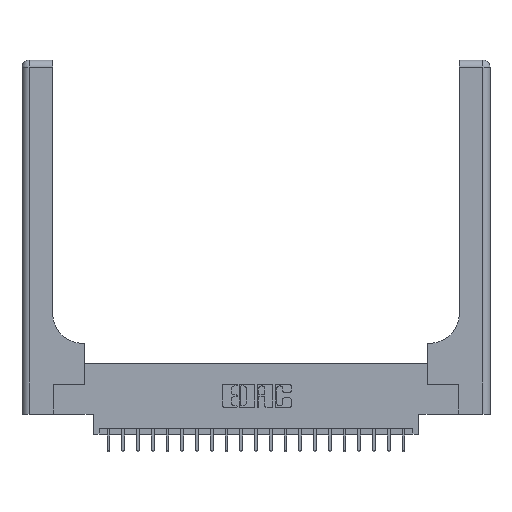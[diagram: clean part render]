
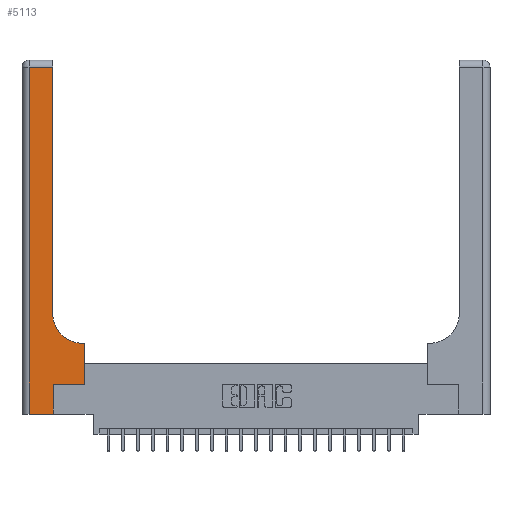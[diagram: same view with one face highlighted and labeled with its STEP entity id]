
A CAD part, top view. The second image highlights one B-rep face of the part: STEP entity #5113.
In plain terms, the highlighted planar face has unit normal (0, 0, 1).
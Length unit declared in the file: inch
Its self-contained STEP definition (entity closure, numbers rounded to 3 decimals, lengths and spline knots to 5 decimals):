
#341 = EDGE_CURVE ( 'NONE', #14062, #20262, #6236, .T. ) ;
#424 = ORIENTED_EDGE ( 'NONE', *, *, #341, .T. ) ;
#533 = LINE ( 'NONE', #12479, #3521 ) ;
#1240 = ORIENTED_EDGE ( 'NONE', *, *, #5312, .T. ) ;
#1293 = DIRECTION ( 'NONE',  ( -1., 0., 0. ) ) ;
#1605 = VECTOR ( 'NONE', #18984, 39.37008 ) ;
#1949 = EDGE_CURVE ( 'NONE', #20262, #14059, #13385, .T. ) ;
#2393 = VERTEX_POINT ( 'NONE', #12320 ) ;
#2599 = VECTOR ( 'NONE', #13983, 39.37008 ) ;
#3425 = ORIENTED_EDGE ( 'NONE', *, *, #14612, .T. ) ;
#3521 = VECTOR ( 'NONE', #17508, 39.37008 ) ;
#3938 = VERTEX_POINT ( 'NONE', #20074 ) ;
#5113 = ADVANCED_FACE ( 'NONE', ( #10994 ), #8161, .F. ) ;
#5312 = EDGE_CURVE ( 'NONE', #14059, #14385, #15191, .T. ) ;
#5616 = CARTESIAN_POINT ( 'NONE',  ( 0.26, 0.85, 0.37 ) ) ;
#6206 = DIRECTION ( 'NONE',  ( 0., -1., 0. ) ) ;
#6236 = LINE ( 'NONE', #7893, #15282 ) ;
#6695 = DIRECTION ( 'NONE',  ( 0., 1., 0. ) ) ;
#7032 = CARTESIAN_POINT ( 'NONE',  ( 0.51, 0.6, 0.37 ) ) ;
#7867 = DIRECTION ( 'NONE',  ( -1., 0., 0. ) ) ;
#7893 = CARTESIAN_POINT ( 'NONE',  ( 0., 2.94, 0.37 ) ) ;
#8161 = PLANE ( 'NONE',  #11349 ) ;
#8549 = CARTESIAN_POINT ( 'NONE',  ( 0.51, 0.85, 0.37 ) ) ;
#8555 = ORIENTED_EDGE ( 'NONE', *, *, #16205, .T. ) ;
#8695 = CARTESIAN_POINT ( 'NONE',  ( 0.528, 0.6, 0.37 ) ) ;
#9153 = LINE ( 'NONE', #20043, #21865 ) ;
#9530 = CARTESIAN_POINT ( 'NONE',  ( 0.06, 2.94, 0.37 ) ) ;
#9998 = LINE ( 'NONE', #15172, #18344 ) ;
#10207 = ORIENTED_EDGE ( 'NONE', *, *, #14818, .T. ) ;
#10309 = DIRECTION ( 'NONE',  ( 1., 0., 0. ) ) ;
#10994 = FACE_OUTER_BOUND ( 'NONE', #13477, .T. ) ;
#11235 = LINE ( 'NONE', #11469, #19562 ) ;
#11349 = AXIS2_PLACEMENT_3D ( 'NONE', #21504, #11626, #1293 ) ;
#11469 = CARTESIAN_POINT ( 'NONE',  ( 0.265, 0.25, 0.37 ) ) ;
#11626 = DIRECTION ( 'NONE',  ( 0., 0., -1. ) ) ;
#12109 = CARTESIAN_POINT ( 'NONE',  ( 0.06, 0., 0.37 ) ) ;
#12320 = CARTESIAN_POINT ( 'NONE',  ( 0.265, 0.25, 0.37 ) ) ;
#12479 = CARTESIAN_POINT ( 'NONE',  ( 0.26, 3., 0.37 ) ) ;
#13316 = ORIENTED_EDGE ( 'NONE', *, *, #17021, .T. ) ;
#13385 = LINE ( 'NONE', #16349, #17826 ) ;
#13477 = EDGE_LOOP ( 'NONE', ( #13316, #424, #16220, #1240, #3425, #8555, #10207, #21589, #15478 ) ) ;
#13983 = DIRECTION ( 'NONE',  ( 1., 0., 0. ) ) ;
#14059 = VERTEX_POINT ( 'NONE', #12109 ) ;
#14062 = VERTEX_POINT ( 'NONE', #17131 ) ;
#14105 = VERTEX_POINT ( 'NONE', #7032 ) ;
#14385 = VERTEX_POINT ( 'NONE', #21178 ) ;
#14612 = EDGE_CURVE ( 'NONE', #14385, #2393, #9998, .T. ) ;
#14818 = EDGE_CURVE ( 'NONE', #3938, #20664, #19136, .T. ) ;
#15172 = CARTESIAN_POINT ( 'NONE',  ( 0.265, 0., 0.37 ) ) ;
#15191 = LINE ( 'NONE', #20591, #2599 ) ;
#15282 = VECTOR ( 'NONE', #7867, 39.37008 ) ;
#15478 = ORIENTED_EDGE ( 'NONE', *, *, #15703, .T. ) ;
#15703 = EDGE_CURVE ( 'NONE', #14105, #16636, #16249, .T. ) ;
#16205 = EDGE_CURVE ( 'NONE', #2393, #3938, #11235, .T. ) ;
#16220 = ORIENTED_EDGE ( 'NONE', *, *, #1949, .T. ) ;
#16249 = CIRCLE ( 'NONE', #17147, 0.25 ) ;
#16349 = CARTESIAN_POINT ( 'NONE',  ( 0.06, 3., 0.37 ) ) ;
#16506 = DIRECTION ( 'NONE',  ( 1., 0., 0. ) ) ;
#16636 = VERTEX_POINT ( 'NONE', #5616 ) ;
#17021 = EDGE_CURVE ( 'NONE', #16636, #14062, #533, .T. ) ;
#17131 = CARTESIAN_POINT ( 'NONE',  ( 0.26, 2.94, 0.37 ) ) ;
#17147 = AXIS2_PLACEMENT_3D ( 'NONE', #8549, #20250, #10309 ) ;
#17332 = CARTESIAN_POINT ( 'NONE',  ( 0.528, 0.25, 0.37 ) ) ;
#17508 = DIRECTION ( 'NONE',  ( 0., 1., 0. ) ) ;
#17826 = VECTOR ( 'NONE', #6206, 39.37008 ) ;
#18344 = VECTOR ( 'NONE', #6695, 39.37008 ) ;
#18409 = DIRECTION ( 'NONE',  ( -1., 0., 0. ) ) ;
#18984 = DIRECTION ( 'NONE',  ( 0., 1., 0. ) ) ;
#19121 = EDGE_CURVE ( 'NONE', #20664, #14105, #9153, .T. ) ;
#19136 = LINE ( 'NONE', #17332, #1605 ) ;
#19562 = VECTOR ( 'NONE', #16506, 39.37008 ) ;
#20043 = CARTESIAN_POINT ( 'NONE',  ( 0.26, 0.6, 0.37 ) ) ;
#20074 = CARTESIAN_POINT ( 'NONE',  ( 0.528, 0.25, 0.37 ) ) ;
#20250 = DIRECTION ( 'NONE',  ( 0., 0., -1. ) ) ;
#20262 = VERTEX_POINT ( 'NONE', #9530 ) ;
#20591 = CARTESIAN_POINT ( 'NONE',  ( 0., 0., 0.37 ) ) ;
#20664 = VERTEX_POINT ( 'NONE', #8695 ) ;
#21178 = CARTESIAN_POINT ( 'NONE',  ( 0.265, 0., 0.37 ) ) ;
#21504 = CARTESIAN_POINT ( 'NONE',  ( 0., 3., 0.37 ) ) ;
#21589 = ORIENTED_EDGE ( 'NONE', *, *, #19121, .T. ) ;
#21865 = VECTOR ( 'NONE', #18409, 39.37008 ) ;
